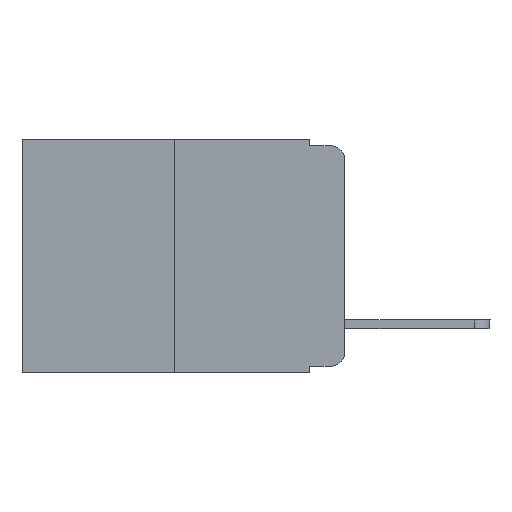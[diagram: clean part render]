
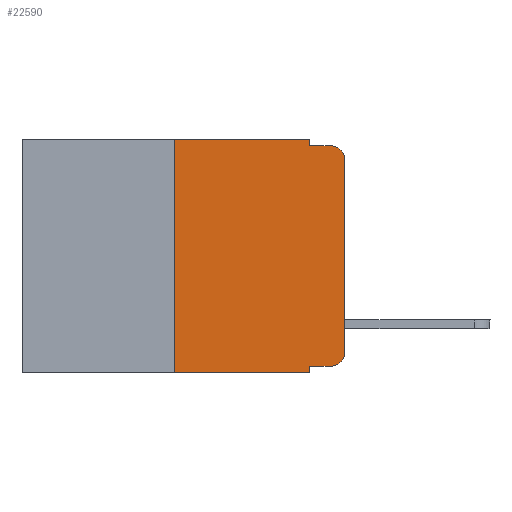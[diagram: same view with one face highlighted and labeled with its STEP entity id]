
A CAD part, left-side view. The second image highlights one B-rep face of the part: STEP entity #22590.
In plain terms, the highlighted planar face has unit normal (-1, 0, 0).
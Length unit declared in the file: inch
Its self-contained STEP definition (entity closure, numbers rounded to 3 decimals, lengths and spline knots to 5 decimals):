
#152 = VERTEX_POINT ( 'NONE', #8805 ) ;
#527 = ORIENTED_EDGE ( 'NONE', *, *, #21523, .F. ) ;
#621 = DIRECTION ( 'NONE',  ( -1., 0., 0. ) ) ;
#684 = EDGE_CURVE ( 'NONE', #18284, #19402, #7108, .T. ) ;
#783 = AXIS2_PLACEMENT_3D ( 'NONE', #6626, #18563, #16628 ) ;
#855 = CARTESIAN_POINT ( 'NONE',  ( 0., 0.051, -0.343 ) ) ;
#1131 = LINE ( 'NONE', #17631, #10011 ) ;
#1292 = LINE ( 'NONE', #4230, #8376 ) ;
#1701 = VERTEX_POINT ( 'NONE', #16102 ) ;
#2656 = VECTOR ( 'NONE', #7752, 39.37008 ) ;
#2664 = VECTOR ( 'NONE', #12423, 39.37008 ) ;
#2988 = LINE ( 'NONE', #14533, #2664 ) ;
#3550 = CARTESIAN_POINT ( 'NONE',  ( 0., 0.25, 0. ) ) ;
#4230 = CARTESIAN_POINT ( 'NONE',  ( 0., 0.051, 0. ) ) ;
#4486 = CARTESIAN_POINT ( 'NONE',  ( 0., 0.02, -0.333 ) ) ;
#5229 = CARTESIAN_POINT ( 'NONE',  ( 0., 0., -0.03 ) ) ;
#5255 = DIRECTION ( 'NONE',  ( 0., 0., 1. ) ) ;
#5290 = CARTESIAN_POINT ( 'NONE',  ( 0., 0.051, 0. ) ) ;
#5731 = CARTESIAN_POINT ( 'NONE',  ( 0., 0.051, -0.01 ) ) ;
#5767 = LINE ( 'NONE', #7215, #6052 ) ;
#5846 = DIRECTION ( 'NONE',  ( 0., -1., 0. ) ) ;
#5977 = VERTEX_POINT ( 'NONE', #3550 ) ;
#6052 = VECTOR ( 'NONE', #20936, 39.37008 ) ;
#6145 = DIRECTION ( 'NONE',  ( 0., 0., -1. ) ) ;
#6245 = ORIENTED_EDGE ( 'NONE', *, *, #17284, .F. ) ;
#6626 = CARTESIAN_POINT ( 'NONE',  ( 0., 0.02, -0.313 ) ) ;
#6653 = CIRCLE ( 'NONE', #783, 0.02 ) ;
#6746 = ORIENTED_EDGE ( 'NONE', *, *, #9526, .T. ) ;
#7108 = LINE ( 'NONE', #11734, #10770 ) ;
#7215 = CARTESIAN_POINT ( 'NONE',  ( 0., 0.25, 0. ) ) ;
#7352 = EDGE_CURVE ( 'NONE', #1701, #8088, #2988, .T. ) ;
#7752 = DIRECTION ( 'NONE',  ( 0., -1., 0. ) ) ;
#7769 = VERTEX_POINT ( 'NONE', #15613 ) ;
#8088 = VERTEX_POINT ( 'NONE', #855 ) ;
#8229 = ORIENTED_EDGE ( 'NONE', *, *, #684, .T. ) ;
#8253 = VERTEX_POINT ( 'NONE', #5229 ) ;
#8376 = VECTOR ( 'NONE', #9860, 39.37008 ) ;
#8393 = EDGE_LOOP ( 'NONE', ( #6746, #14303, #15697, #16334, #12320, #527, #11642, #6245, #8229, #21918 ) ) ;
#8529 = VERTEX_POINT ( 'NONE', #5731 ) ;
#8805 = CARTESIAN_POINT ( 'NONE',  ( 0., 0., -0.313 ) ) ;
#9526 = EDGE_CURVE ( 'NONE', #152, #8253, #18443, .T. ) ;
#9849 = EDGE_CURVE ( 'NONE', #13882, #8529, #1292, .T. ) ;
#9860 = DIRECTION ( 'NONE',  ( 0., 0., -1. ) ) ;
#10011 = VECTOR ( 'NONE', #17538, 39.37008 ) ;
#10770 = VECTOR ( 'NONE', #5846, 39.37008 ) ;
#11642 = ORIENTED_EDGE ( 'NONE', *, *, #7352, .T. ) ;
#11734 = CARTESIAN_POINT ( 'NONE',  ( 0., 0.051, -0.333 ) ) ;
#12199 = PLANE ( 'NONE',  #16746 ) ;
#12319 = CARTESIAN_POINT ( 'NONE',  ( 0., 0.02, -0.03 ) ) ;
#12320 = ORIENTED_EDGE ( 'NONE', *, *, #22080, .F. ) ;
#12423 = DIRECTION ( 'NONE',  ( 0., -1., 0. ) ) ;
#12972 = VECTOR ( 'NONE', #16116, 39.37008 ) ;
#13882 = VERTEX_POINT ( 'NONE', #5290 ) ;
#14303 = ORIENTED_EDGE ( 'NONE', *, *, #15968, .T. ) ;
#14524 = FACE_OUTER_BOUND ( 'NONE', #8393, .T. ) ;
#14533 = CARTESIAN_POINT ( 'NONE',  ( 0., 0.473, -0.343 ) ) ;
#15065 = LINE ( 'NONE', #23823, #12972 ) ;
#15613 = CARTESIAN_POINT ( 'NONE',  ( 0., 0.02, -0.01 ) ) ;
#15697 = ORIENTED_EDGE ( 'NONE', *, *, #22209, .F. ) ;
#15927 = DIRECTION ( 'NONE',  ( 1., 0., 0. ) ) ;
#15968 = EDGE_CURVE ( 'NONE', #8253, #7769, #16130, .T. ) ;
#16102 = CARTESIAN_POINT ( 'NONE',  ( 0., 0.25, -0.343 ) ) ;
#16116 = DIRECTION ( 'NONE',  ( 0., 0., -1. ) ) ;
#16130 = CIRCLE ( 'NONE', #18963, 0.02 ) ;
#16334 = ORIENTED_EDGE ( 'NONE', *, *, #9849, .F. ) ;
#16449 = EDGE_CURVE ( 'NONE', #19402, #152, #6653, .T. ) ;
#16628 = DIRECTION ( 'NONE',  ( 0., 0., -1. ) ) ;
#16746 = AXIS2_PLACEMENT_3D ( 'NONE', #21931, #15927, #6145 ) ;
#16822 = CARTESIAN_POINT ( 'NONE',  ( 0., 0., 0. ) ) ;
#16880 = VECTOR ( 'NONE', #5255, 39.37008 ) ;
#16960 = CARTESIAN_POINT ( 'NONE',  ( 0., 0.051, -0.333 ) ) ;
#17284 = EDGE_CURVE ( 'NONE', #18284, #8088, #15065, .T. ) ;
#17439 = CARTESIAN_POINT ( 'NONE',  ( 0., 0.051, -0.01 ) ) ;
#17538 = DIRECTION ( 'NONE',  ( 0., -1., 0. ) ) ;
#17631 = CARTESIAN_POINT ( 'NONE',  ( 0., 0.473, 0. ) ) ;
#18284 = VERTEX_POINT ( 'NONE', #16960 ) ;
#18443 = LINE ( 'NONE', #16822, #16880 ) ;
#18563 = DIRECTION ( 'NONE',  ( -1., 0., 0. ) ) ;
#18963 = AXIS2_PLACEMENT_3D ( 'NONE', #12319, #621, #22136 ) ;
#19402 = VERTEX_POINT ( 'NONE', #4486 ) ;
#20936 = DIRECTION ( 'NONE',  ( 0., 0., 1. ) ) ;
#21523 = EDGE_CURVE ( 'NONE', #1701, #5977, #5767, .T. ) ;
#21918 = ORIENTED_EDGE ( 'NONE', *, *, #16449, .T. ) ;
#21931 = CARTESIAN_POINT ( 'NONE',  ( 0., 0.473, 0. ) ) ;
#22080 = EDGE_CURVE ( 'NONE', #5977, #13882, #1131, .T. ) ;
#22136 = DIRECTION ( 'NONE',  ( 0., 0., -1. ) ) ;
#22209 = EDGE_CURVE ( 'NONE', #8529, #7769, #23745, .T. ) ;
#22590 = ADVANCED_FACE ( 'NONE', ( #14524 ), #12199, .F. ) ;
#23745 = LINE ( 'NONE', #17439, #2656 ) ;
#23823 = CARTESIAN_POINT ( 'NONE',  ( 0., 0.051, 0. ) ) ;
